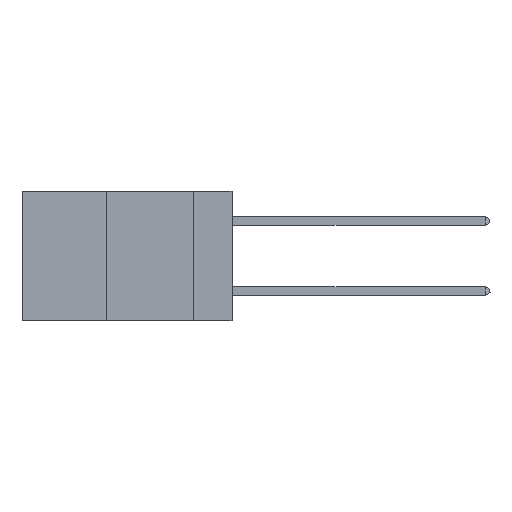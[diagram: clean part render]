
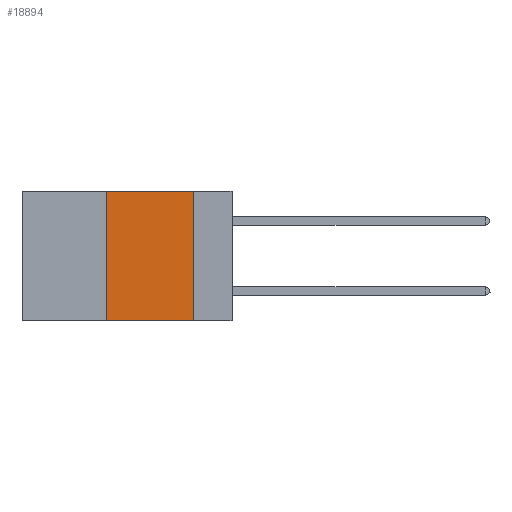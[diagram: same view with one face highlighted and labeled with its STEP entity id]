
A CAD part, left-side view. The second image highlights one B-rep face of the part: STEP entity #18894.
In plain terms, the highlighted planar face has unit normal (-1, 0, 0).
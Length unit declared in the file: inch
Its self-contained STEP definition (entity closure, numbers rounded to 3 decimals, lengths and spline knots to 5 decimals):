
#193 = VERTEX_POINT ( 'NONE', #22475 ) ;
#1534 = VERTEX_POINT ( 'NONE', #13948 ) ;
#3461 = DIRECTION ( 'NONE',  ( 1., 0., 0. ) ) ;
#3839 = LINE ( 'NONE', #23982, #28285 ) ;
#4944 = LINE ( 'NONE', #16843, #30174 ) ;
#6054 = VERTEX_POINT ( 'NONE', #7799 ) ;
#6903 = VECTOR ( 'NONE', #9117, 39.37008 ) ;
#7799 = CARTESIAN_POINT ( 'NONE',  ( 0., 0.36, -0.37 ) ) ;
#9117 = DIRECTION ( 'NONE',  ( 0., -1., 0. ) ) ;
#9507 = EDGE_CURVE ( 'NONE', #193, #1534, #3839, .T. ) ;
#9557 = EDGE_CURVE ( 'NONE', #6054, #1534, #27143, .T. ) ;
#9775 = DIRECTION ( 'NONE',  ( 0., -1., 0. ) ) ;
#10903 = CARTESIAN_POINT ( 'NONE',  ( 0., 0.36, 0. ) ) ;
#10932 = ORIENTED_EDGE ( 'NONE', *, *, #9507, .F. ) ;
#13261 = VECTOR ( 'NONE', #31266, 39.37008 ) ;
#13532 = EDGE_CURVE ( 'NONE', #6054, #26985, #15952, .T. ) ;
#13588 = ORIENTED_EDGE ( 'NONE', *, *, #13532, .F. ) ;
#13948 = CARTESIAN_POINT ( 'NONE',  ( 0., 0.11, -0.37 ) ) ;
#14363 = ORIENTED_EDGE ( 'NONE', *, *, #9557, .T. ) ;
#15762 = AXIS2_PLACEMENT_3D ( 'NONE', #22597, #3461, #20379 ) ;
#15952 = LINE ( 'NONE', #21506, #13261 ) ;
#16843 = CARTESIAN_POINT ( 'NONE',  ( 0., 0.6, 0. ) ) ;
#18894 = ADVANCED_FACE ( 'NONE', ( #23308 ), #29831, .F. ) ;
#19073 = CARTESIAN_POINT ( 'NONE',  ( 0., 0.6, -0.37 ) ) ;
#19337 = EDGE_CURVE ( 'NONE', #26985, #193, #4944, .T. ) ;
#20379 = DIRECTION ( 'NONE',  ( 0., 0., -1. ) ) ;
#21506 = CARTESIAN_POINT ( 'NONE',  ( 0., 0.36, 0. ) ) ;
#22475 = CARTESIAN_POINT ( 'NONE',  ( 0., 0.11, 0. ) ) ;
#22597 = CARTESIAN_POINT ( 'NONE',  ( 0., 0.6, 0. ) ) ;
#23308 = FACE_OUTER_BOUND ( 'NONE', #27547, .T. ) ;
#23982 = CARTESIAN_POINT ( 'NONE',  ( 0., 0.11, 0. ) ) ;
#24082 = DIRECTION ( 'NONE',  ( 0., 0., -1. ) ) ;
#26985 = VERTEX_POINT ( 'NONE', #10903 ) ;
#27143 = LINE ( 'NONE', #19073, #6903 ) ;
#27547 = EDGE_LOOP ( 'NONE', ( #10932, #27589, #13588, #14363 ) ) ;
#27589 = ORIENTED_EDGE ( 'NONE', *, *, #19337, .F. ) ;
#28285 = VECTOR ( 'NONE', #24082, 39.37008 ) ;
#29831 = PLANE ( 'NONE',  #15762 ) ;
#30174 = VECTOR ( 'NONE', #9775, 39.37008 ) ;
#31266 = DIRECTION ( 'NONE',  ( 0., 0., 1. ) ) ;
